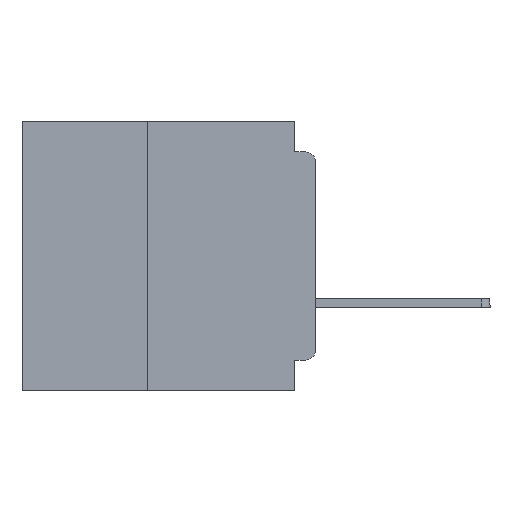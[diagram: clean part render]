
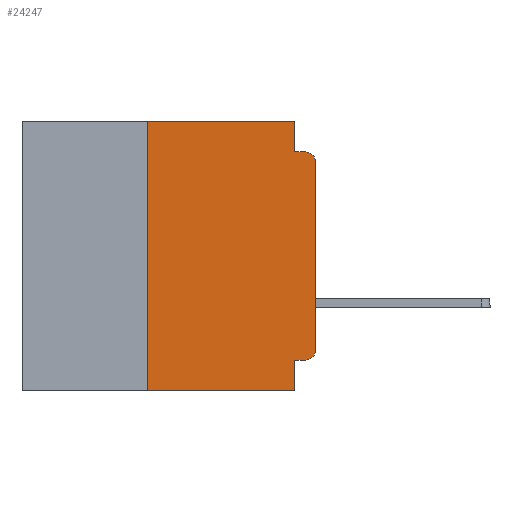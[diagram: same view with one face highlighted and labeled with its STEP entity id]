
A CAD part, left-side view. The second image highlights one B-rep face of the part: STEP entity #24247.
In plain terms, the highlighted planar face has unit normal (-1, 0, 0).
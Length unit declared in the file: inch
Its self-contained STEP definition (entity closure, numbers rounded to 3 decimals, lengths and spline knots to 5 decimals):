
#102 = LINE ( 'NONE', #35976, #13682 ) ;
#129 = DIRECTION ( 'NONE',  ( 0., -1., 0. ) ) ;
#614 = DIRECTION ( 'NONE',  ( 0., 0., 1. ) ) ;
#1864 = EDGE_LOOP ( 'NONE', ( #51040, #39188, #3672, #17198, #18756, #10087, #36831, #51862, #55062, #62960 ) ) ;
#2290 = VERTEX_POINT ( 'NONE', #46258 ) ;
#3672 = ORIENTED_EDGE ( 'NONE', *, *, #49489, .F. ) ;
#4416 = DIRECTION ( 'NONE',  ( 0., 0., -1. ) ) ;
#5470 = VERTEX_POINT ( 'NONE', #37365 ) ;
#6095 = AXIS2_PLACEMENT_3D ( 'NONE', #40678, #10521, #45759 ) ;
#6984 = CARTESIAN_POINT ( 'NONE',  ( 0., 0.031, 0. ) ) ;
#8878 = CARTESIAN_POINT ( 'NONE',  ( 0., 0.437, 0. ) ) ;
#10087 = ORIENTED_EDGE ( 'NONE', *, *, #34321, .F. ) ;
#10424 = CARTESIAN_POINT ( 'NONE',  ( 0., 0.437, -0.4 ) ) ;
#10521 = DIRECTION ( 'NONE',  ( -1., 0., 0. ) ) ;
#10742 = DIRECTION ( 'NONE',  ( 0., -1., 0. ) ) ;
#12310 = VECTOR ( 'NONE', #30717, 39.37008 ) ;
#13010 = VECTOR ( 'NONE', #129, 39.37008 ) ;
#13282 = LINE ( 'NONE', #57017, #65366 ) ;
#13682 = VECTOR ( 'NONE', #614, 39.37008 ) ;
#14605 = LINE ( 'NONE', #10424, #13010 ) ;
#16063 = VERTEX_POINT ( 'NONE', #33908 ) ;
#17198 = ORIENTED_EDGE ( 'NONE', *, *, #63708, .F. ) ;
#17490 = VECTOR ( 'NONE', #51892, 39.37008 ) ;
#18756 = ORIENTED_EDGE ( 'NONE', *, *, #30962, .F. ) ;
#19543 = CARTESIAN_POINT ( 'NONE',  ( 0., 0.25, -0.4 ) ) ;
#21991 = VECTOR ( 'NONE', #10742, 39.37008 ) ;
#24136 = DIRECTION ( 'NONE',  ( 1., 0., 0. ) ) ;
#24247 = ADVANCED_FACE ( 'NONE', ( #54471 ), #44136, .F. ) ;
#25998 = CARTESIAN_POINT ( 'NONE',  ( 0., 0., -0.045 ) ) ;
#26472 = EDGE_CURVE ( 'NONE', #45753, #16063, #49338, .T. ) ;
#26676 = CARTESIAN_POINT ( 'NONE',  ( 0., 0.25, 0. ) ) ;
#26860 = DIRECTION ( 'NONE',  ( 0., -1., 0. ) ) ;
#29428 = VERTEX_POINT ( 'NONE', #52851 ) ;
#30573 = CARTESIAN_POINT ( 'NONE',  ( 0., 0.031, -0.045 ) ) ;
#30717 = DIRECTION ( 'NONE',  ( 0., 0., 1. ) ) ;
#30962 = EDGE_CURVE ( 'NONE', #42005, #39078, #13282, .T. ) ;
#32414 = LINE ( 'NONE', #46806, #17490 ) ;
#33908 = CARTESIAN_POINT ( 'NONE',  ( 0., 0., -0.06 ) ) ;
#34321 = EDGE_CURVE ( 'NONE', #62183, #42005, #102, .T. ) ;
#34679 = DIRECTION ( 'NONE',  ( -1., 0., 0. ) ) ;
#35478 = CARTESIAN_POINT ( 'NONE',  ( 0., 0.031, -0.4 ) ) ;
#35976 = CARTESIAN_POINT ( 'NONE',  ( 0., 0.25, -0.4 ) ) ;
#36430 = VECTOR ( 'NONE', #55994, 39.37008 ) ;
#36831 = ORIENTED_EDGE ( 'NONE', *, *, #38244, .T. ) ;
#36875 = LINE ( 'NONE', #25998, #21991 ) ;
#37365 = CARTESIAN_POINT ( 'NONE',  ( 0., 0.031, -0.355 ) ) ;
#38244 = EDGE_CURVE ( 'NONE', #62183, #2290, #14605, .T. ) ;
#39078 = VERTEX_POINT ( 'NONE', #6984 ) ;
#39188 = ORIENTED_EDGE ( 'NONE', *, *, #42315, .T. ) ;
#39336 = EDGE_CURVE ( 'NONE', #29428, #45753, #53176, .T. ) ;
#40533 = DIRECTION ( 'NONE',  ( 0., 0., -1. ) ) ;
#40678 = CARTESIAN_POINT ( 'NONE',  ( 0., 0.015, -0.06 ) ) ;
#40717 = CARTESIAN_POINT ( 'NONE',  ( 0., 0., -0.355 ) ) ;
#41009 = VECTOR ( 'NONE', #40533, 39.37008 ) ;
#42005 = VERTEX_POINT ( 'NONE', #26676 ) ;
#42315 = EDGE_CURVE ( 'NONE', #16063, #42618, #45636, .T. ) ;
#42595 = LINE ( 'NONE', #35478, #41009 ) ;
#42618 = VERTEX_POINT ( 'NONE', #48387 ) ;
#44136 = PLANE ( 'NONE',  #64395 ) ;
#45636 = CIRCLE ( 'NONE', #6095, 0.015 ) ;
#45753 = VERTEX_POINT ( 'NONE', #52434 ) ;
#45759 = DIRECTION ( 'NONE',  ( 0., 0., -1. ) ) ;
#46258 = CARTESIAN_POINT ( 'NONE',  ( 0., 0.031, -0.4 ) ) ;
#46806 = CARTESIAN_POINT ( 'NONE',  ( 0., 0.031, 0. ) ) ;
#48387 = CARTESIAN_POINT ( 'NONE',  ( 0., 0.015, -0.045 ) ) ;
#49338 = LINE ( 'NONE', #60913, #12310 ) ;
#49489 = EDGE_CURVE ( 'NONE', #54289, #42618, #36875, .T. ) ;
#49885 = LINE ( 'NONE', #40717, #36430 ) ;
#50357 = AXIS2_PLACEMENT_3D ( 'NONE', #64917, #34679, #4416 ) ;
#51040 = ORIENTED_EDGE ( 'NONE', *, *, #26472, .T. ) ;
#51862 = ORIENTED_EDGE ( 'NONE', *, *, #60015, .F. ) ;
#51892 = DIRECTION ( 'NONE',  ( 0., 0., -1. ) ) ;
#52434 = CARTESIAN_POINT ( 'NONE',  ( 0., 0., -0.34 ) ) ;
#52851 = CARTESIAN_POINT ( 'NONE',  ( 0., 0.015, -0.355 ) ) ;
#53176 = CIRCLE ( 'NONE', #50357, 0.015 ) ;
#54289 = VERTEX_POINT ( 'NONE', #30573 ) ;
#54471 = FACE_OUTER_BOUND ( 'NONE', #1864, .T. ) ;
#55062 = ORIENTED_EDGE ( 'NONE', *, *, #62946, .F. ) ;
#55994 = DIRECTION ( 'NONE',  ( 0., 1., 0. ) ) ;
#57017 = CARTESIAN_POINT ( 'NONE',  ( 0., 0.437, 0. ) ) ;
#59376 = DIRECTION ( 'NONE',  ( 0., 0., -1. ) ) ;
#60015 = EDGE_CURVE ( 'NONE', #5470, #2290, #42595, .T. ) ;
#60913 = CARTESIAN_POINT ( 'NONE',  ( 0., 0., 0. ) ) ;
#62183 = VERTEX_POINT ( 'NONE', #19543 ) ;
#62946 = EDGE_CURVE ( 'NONE', #29428, #5470, #49885, .T. ) ;
#62960 = ORIENTED_EDGE ( 'NONE', *, *, #39336, .T. ) ;
#63708 = EDGE_CURVE ( 'NONE', #39078, #54289, #32414, .T. ) ;
#64395 = AXIS2_PLACEMENT_3D ( 'NONE', #8878, #24136, #59376 ) ;
#64917 = CARTESIAN_POINT ( 'NONE',  ( 0., 0.015, -0.34 ) ) ;
#65366 = VECTOR ( 'NONE', #26860, 39.37008 ) ;
